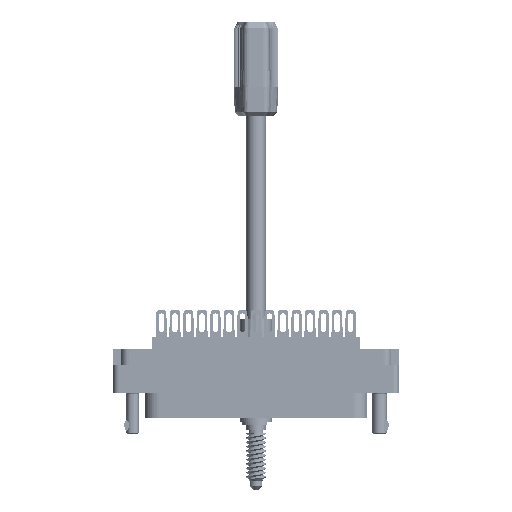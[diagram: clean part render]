
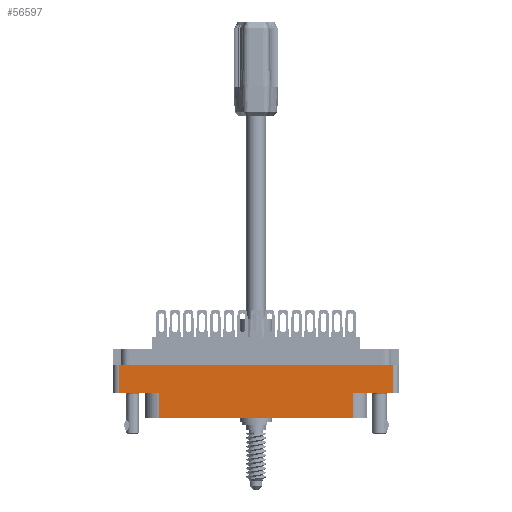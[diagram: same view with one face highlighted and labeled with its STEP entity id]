
A CAD part, front view. The second image highlights one B-rep face of the part: STEP entity #56597.
In plain terms, the highlighted planar face has unit normal (0, -1, 0).
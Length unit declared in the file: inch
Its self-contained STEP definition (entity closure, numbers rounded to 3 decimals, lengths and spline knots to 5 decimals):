
#250 = VERTEX_POINT ( 'NONE', #99358 ) ;
#1355 = FACE_OUTER_BOUND ( 'NONE', #87444, .T. ) ;
#5848 = CARTESIAN_POINT ( 'NONE',  ( 0.9315, -0.7625, -0.54 ) ) ;
#7304 = LINE ( 'NONE', #81440, #40158 ) ;
#7759 = LINE ( 'NONE', #25770, #98337 ) ;
#11462 = ORIENTED_EDGE ( 'NONE', *, *, #91099, .F. ) ;
#12484 = ORIENTED_EDGE ( 'NONE', *, *, #78674, .T. ) ;
#12872 = DIRECTION ( 'NONE',  ( 0., -1., 0. ) ) ;
#13156 = DIRECTION ( 'NONE',  ( 0., 0., 1. ) ) ;
#13918 = CARTESIAN_POINT ( 'NONE',  ( 1.313, -0.7625, -0.78 ) ) ;
#17805 = CARTESIAN_POINT ( 'NONE',  ( -1.313, -0.7625, -0.54 ) ) ;
#18937 = LINE ( 'NONE', #41525, #102732 ) ;
#22124 = VECTOR ( 'NONE', #88302, 39.37008 ) ;
#22410 = DIRECTION ( 'NONE',  ( 0., 0., -1. ) ) ;
#22470 = PLANE ( 'NONE',  #55594 ) ;
#24070 = LINE ( 'NONE', #38109, #65288 ) ;
#24354 = VERTEX_POINT ( 'NONE', #103989 ) ;
#25770 = CARTESIAN_POINT ( 'NONE',  ( -1.313, -0.7625, -0.78 ) ) ;
#26810 = ORIENTED_EDGE ( 'NONE', *, *, #112540, .T. ) ;
#28371 = EDGE_CURVE ( 'NONE', #80993, #80854, #76275, .T. ) ;
#30632 = ORIENTED_EDGE ( 'NONE', *, *, #28371, .T. ) ;
#38109 = CARTESIAN_POINT ( 'NONE',  ( 0., -0.7625, -0.54 ) ) ;
#38484 = DIRECTION ( 'NONE',  ( 1., 0., 0. ) ) ;
#40158 = VECTOR ( 'NONE', #53917, 39.37008 ) ;
#41525 = CARTESIAN_POINT ( 'NONE',  ( 0., -0.7625, -0.274 ) ) ;
#53917 = DIRECTION ( 'NONE',  ( 1., 0., 0. ) ) ;
#55437 = EDGE_CURVE ( 'NONE', #250, #102126, #104486, .T. ) ;
#55594 = AXIS2_PLACEMENT_3D ( 'NONE', #83796, #12872, #110333 ) ;
#56597 = ADVANCED_FACE ( 'NONE', ( #1355 ), #22470, .T. ) ;
#60383 = CARTESIAN_POINT ( 'NONE',  ( -1.313, -0.7625, -0.274 ) ) ;
#65288 = VECTOR ( 'NONE', #38484, 39.37008 ) ;
#70713 = CARTESIAN_POINT ( 'NONE',  ( 0.9315, -0.7625, -0.54 ) ) ;
#72193 = CARTESIAN_POINT ( 'NONE',  ( 0., -0.7625, -0.54 ) ) ;
#73285 = ORIENTED_EDGE ( 'NONE', *, *, #73631, .T. ) ;
#73383 = VERTEX_POINT ( 'NONE', #17805 ) ;
#73526 = CARTESIAN_POINT ( 'NONE',  ( -0.9315, -0.7625, -0.78 ) ) ;
#73631 = EDGE_CURVE ( 'NONE', #80854, #250, #7304, .T. ) ;
#73717 = CARTESIAN_POINT ( 'NONE',  ( 1.313, -0.7625, -0.274 ) ) ;
#75047 = CARTESIAN_POINT ( 'NONE',  ( -0.9315, -0.7625, -0.54 ) ) ;
#75823 = ORIENTED_EDGE ( 'NONE', *, *, #55437, .T. ) ;
#76275 = LINE ( 'NONE', #110279, #98239 ) ;
#76681 = VERTEX_POINT ( 'NONE', #73717 ) ;
#78674 = EDGE_CURVE ( 'NONE', #112355, #73383, #7759, .T. ) ;
#80854 = VERTEX_POINT ( 'NONE', #73526 ) ;
#80993 = VERTEX_POINT ( 'NONE', #75047 ) ;
#81440 = CARTESIAN_POINT ( 'NONE',  ( -1.375, -0.7625, -0.78 ) ) ;
#83346 = VECTOR ( 'NONE', #106680, 39.37008 ) ;
#83796 = CARTESIAN_POINT ( 'NONE',  ( -1.375, -0.7625, -0.78 ) ) ;
#84517 = DIRECTION ( 'NONE',  ( 1., 0., 0. ) ) ;
#86697 = ORIENTED_EDGE ( 'NONE', *, *, #104234, .F. ) ;
#87337 = EDGE_CURVE ( 'NONE', #24354, #76681, #107430, .T. ) ;
#87444 = EDGE_LOOP ( 'NONE', ( #11462, #12484, #26810, #30632, #73285, #75823, #86697, #105305 ) ) ;
#88302 = DIRECTION ( 'NONE',  ( 0., 0., 1. ) ) ;
#90170 = LINE ( 'NONE', #72193, #83346 ) ;
#91099 = EDGE_CURVE ( 'NONE', #112355, #76681, #18937, .T. ) ;
#98239 = VECTOR ( 'NONE', #22410, 39.37008 ) ;
#98337 = VECTOR ( 'NONE', #112556, 39.37008 ) ;
#99358 = CARTESIAN_POINT ( 'NONE',  ( 0.9315, -0.7625, -0.78 ) ) ;
#102126 = VERTEX_POINT ( 'NONE', #5848 ) ;
#102732 = VECTOR ( 'NONE', #84517, 39.37008 ) ;
#103989 = CARTESIAN_POINT ( 'NONE',  ( 1.313, -0.7625, -0.54 ) ) ;
#104234 = EDGE_CURVE ( 'NONE', #24354, #102126, #90170, .T. ) ;
#104486 = LINE ( 'NONE', #70713, #22124 ) ;
#104711 = VECTOR ( 'NONE', #13156, 39.37008 ) ;
#105305 = ORIENTED_EDGE ( 'NONE', *, *, #87337, .T. ) ;
#106680 = DIRECTION ( 'NONE',  ( -1., 0., 0. ) ) ;
#107430 = LINE ( 'NONE', #13918, #104711 ) ;
#110279 = CARTESIAN_POINT ( 'NONE',  ( -0.9315, -0.7625, -0.78 ) ) ;
#110333 = DIRECTION ( 'NONE',  ( 0., 0., -1. ) ) ;
#112355 = VERTEX_POINT ( 'NONE', #60383 ) ;
#112540 = EDGE_CURVE ( 'NONE', #73383, #80993, #24070, .T. ) ;
#112556 = DIRECTION ( 'NONE',  ( 0., 0., -1. ) ) ;
